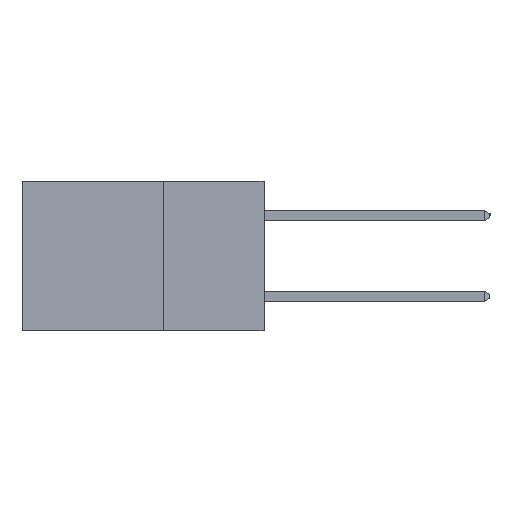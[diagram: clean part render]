
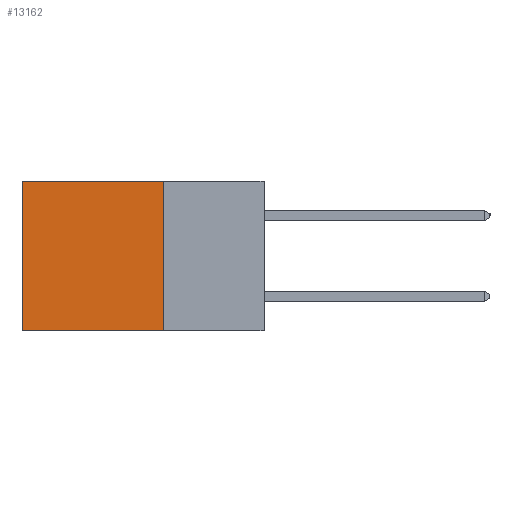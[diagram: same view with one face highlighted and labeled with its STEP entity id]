
A CAD part, left-side view. The second image highlights one B-rep face of the part: STEP entity #13162.
In plain terms, the highlighted planar face has unit normal (-1, 0, 0).
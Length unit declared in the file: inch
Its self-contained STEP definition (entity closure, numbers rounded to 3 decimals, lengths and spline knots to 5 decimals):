
#87 = CARTESIAN_POINT ( 'NONE',  ( 0.2615, 0.25, 0. ) ) ;
#126 = CARTESIAN_POINT ( 'NONE',  ( 0.2615, 0.25, -0.37 ) ) ;
#134 = VERTEX_POINT ( 'NONE', #87 ) ;
#577 = DIRECTION ( 'NONE',  ( 0., 1., 0. ) ) ;
#1464 = EDGE_LOOP ( 'NONE', ( #16997, #16113, #10736, #3116 ) ) ;
#1537 = PLANE ( 'NONE',  #7673 ) ;
#2014 = VERTEX_POINT ( 'NONE', #16262 ) ;
#2072 = CARTESIAN_POINT ( 'NONE',  ( 0.2615, 0.25, 0. ) ) ;
#2543 = CARTESIAN_POINT ( 'NONE',  ( 0.2615, 0.25, -0.37 ) ) ;
#3020 = CARTESIAN_POINT ( 'NONE',  ( 0.2615, 0.6, -0.37 ) ) ;
#3116 = ORIENTED_EDGE ( 'NONE', *, *, #11410, .T. ) ;
#4334 = EDGE_CURVE ( 'NONE', #134, #9748, #12479, .T. ) ;
#5265 = LINE ( 'NONE', #2072, #5321 ) ;
#5321 = VECTOR ( 'NONE', #577, 39.37008 ) ;
#7215 = VECTOR ( 'NONE', #12760, 39.37008 ) ;
#7472 = EDGE_CURVE ( 'NONE', #2014, #11242, #14594, .T. ) ;
#7673 = AXIS2_PLACEMENT_3D ( 'NONE', #126, #8826, #14166 ) ;
#8807 = DIRECTION ( 'NONE',  ( 0., 0., -1. ) ) ;
#8826 = DIRECTION ( 'NONE',  ( 1., 0., 0. ) ) ;
#9748 = VERTEX_POINT ( 'NONE', #2543 ) ;
#10023 = CARTESIAN_POINT ( 'NONE',  ( 0.2615, 0.6, -0.37 ) ) ;
#10736 = ORIENTED_EDGE ( 'NONE', *, *, #4334, .F. ) ;
#11242 = VERTEX_POINT ( 'NONE', #3020 ) ;
#11410 = EDGE_CURVE ( 'NONE', #134, #2014, #5265, .T. ) ;
#11818 = VECTOR ( 'NONE', #8807, 39.37008 ) ;
#12479 = LINE ( 'NONE', #14168, #7215 ) ;
#12544 = CARTESIAN_POINT ( 'NONE',  ( 0.2615, 0.25, -0.37 ) ) ;
#12760 = DIRECTION ( 'NONE',  ( 0., 0., -1. ) ) ;
#13040 = FACE_OUTER_BOUND ( 'NONE', #1464, .T. ) ;
#13162 = ADVANCED_FACE ( 'NONE', ( #13040 ), #1537, .F. ) ;
#14166 = DIRECTION ( 'NONE',  ( 0., 0., -1. ) ) ;
#14168 = CARTESIAN_POINT ( 'NONE',  ( 0.2615, 0.25, -0.37 ) ) ;
#14330 = LINE ( 'NONE', #12544, #15000 ) ;
#14513 = EDGE_CURVE ( 'NONE', #9748, #11242, #14330, .T. ) ;
#14594 = LINE ( 'NONE', #10023, #11818 ) ;
#15000 = VECTOR ( 'NONE', #15448, 39.37008 ) ;
#15448 = DIRECTION ( 'NONE',  ( 0., 1., 0. ) ) ;
#16113 = ORIENTED_EDGE ( 'NONE', *, *, #14513, .F. ) ;
#16262 = CARTESIAN_POINT ( 'NONE',  ( 0.2615, 0.6, 0. ) ) ;
#16997 = ORIENTED_EDGE ( 'NONE', *, *, #7472, .T. ) ;
